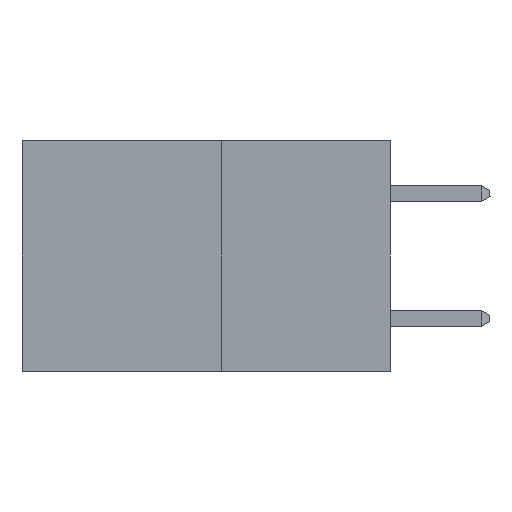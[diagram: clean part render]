
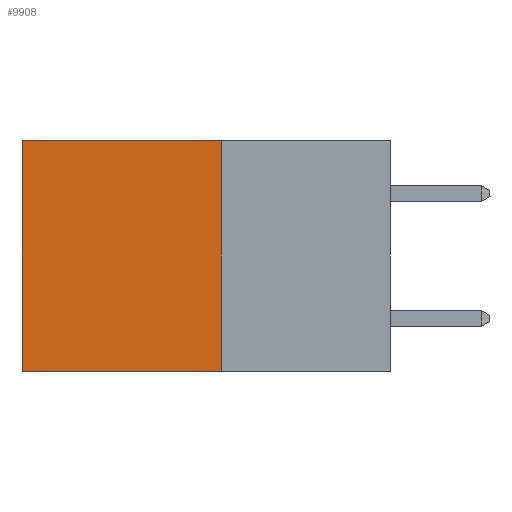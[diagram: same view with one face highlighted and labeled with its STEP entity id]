
A CAD part, left-side view. The second image highlights one B-rep face of the part: STEP entity #9908.
In plain terms, the highlighted planar face has unit normal (-1, 0, 0).
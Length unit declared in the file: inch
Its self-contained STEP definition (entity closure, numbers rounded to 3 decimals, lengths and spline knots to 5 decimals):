
#22 = ORIENTED_EDGE ( 'NONE', *, *, #6897, .T. ) ;
#521 = VERTEX_POINT ( 'NONE', #6526 ) ;
#938 = CARTESIAN_POINT ( 'NONE',  ( 0.277, 0.27, -0.37 ) ) ;
#1564 = LINE ( 'NONE', #6733, #5322 ) ;
#3171 = DIRECTION ( 'NONE',  ( 0., 0., -1. ) ) ;
#3219 = CARTESIAN_POINT ( 'NONE',  ( 0.277, 0.59, -0.37 ) ) ;
#5322 = VECTOR ( 'NONE', #6980, 39.37008 ) ;
#5325 = EDGE_LOOP ( 'NONE', ( #13835, #14782, #15252, #22 ) ) ;
#6460 = CARTESIAN_POINT ( 'NONE',  ( 0.277, 0.27, 0. ) ) ;
#6526 = CARTESIAN_POINT ( 'NONE',  ( 0.277, 0.59, 0. ) ) ;
#6546 = DIRECTION ( 'NONE',  ( 0., 1., 0. ) ) ;
#6696 = VECTOR ( 'NONE', #3171, 39.37008 ) ;
#6733 = CARTESIAN_POINT ( 'NONE',  ( 0.277, 0.27, -0.37 ) ) ;
#6861 = AXIS2_PLACEMENT_3D ( 'NONE', #938, #14240, #19713 ) ;
#6897 = EDGE_CURVE ( 'NONE', #12105, #521, #10254, .T. ) ;
#6980 = DIRECTION ( 'NONE',  ( 0., 1., 0. ) ) ;
#8137 = EDGE_CURVE ( 'NONE', #521, #16539, #18912, .T. ) ;
#8449 = CARTESIAN_POINT ( 'NONE',  ( 0.277, 0.27, -0.37 ) ) ;
#9037 = DIRECTION ( 'NONE',  ( 0., 0., -1. ) ) ;
#9900 = VECTOR ( 'NONE', #9037, 39.37008 ) ;
#9908 = ADVANCED_FACE ( 'NONE', ( #18835 ), #12129, .F. ) ;
#10254 = LINE ( 'NONE', #6460, #18199 ) ;
#11238 = EDGE_CURVE ( 'NONE', #19937, #16539, #1564, .T. ) ;
#11449 = EDGE_CURVE ( 'NONE', #12105, #19937, #13915, .T. ) ;
#12105 = VERTEX_POINT ( 'NONE', #19736 ) ;
#12129 = PLANE ( 'NONE',  #6861 ) ;
#13835 = ORIENTED_EDGE ( 'NONE', *, *, #8137, .T. ) ;
#13915 = LINE ( 'NONE', #8449, #9900 ) ;
#14240 = DIRECTION ( 'NONE',  ( 1., 0., 0. ) ) ;
#14782 = ORIENTED_EDGE ( 'NONE', *, *, #11238, .F. ) ;
#15252 = ORIENTED_EDGE ( 'NONE', *, *, #11449, .F. ) ;
#16539 = VERTEX_POINT ( 'NONE', #18072 ) ;
#18072 = CARTESIAN_POINT ( 'NONE',  ( 0.277, 0.59, -0.37 ) ) ;
#18199 = VECTOR ( 'NONE', #6546, 39.37008 ) ;
#18835 = FACE_OUTER_BOUND ( 'NONE', #5325, .T. ) ;
#18912 = LINE ( 'NONE', #3219, #6696 ) ;
#19713 = DIRECTION ( 'NONE',  ( 0., 0., -1. ) ) ;
#19736 = CARTESIAN_POINT ( 'NONE',  ( 0.277, 0.27, 0. ) ) ;
#19926 = CARTESIAN_POINT ( 'NONE',  ( 0.277, 0.27, -0.37 ) ) ;
#19937 = VERTEX_POINT ( 'NONE', #19926 ) ;
